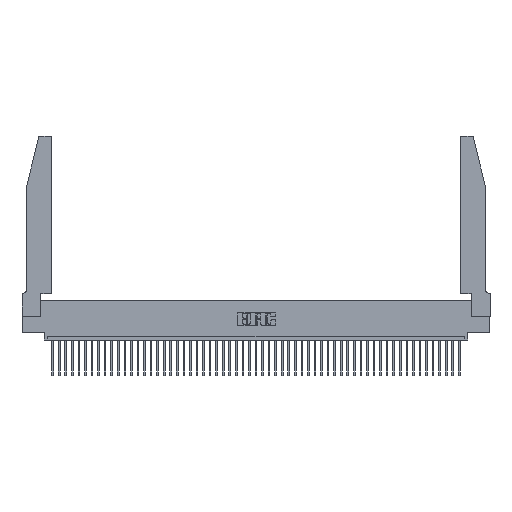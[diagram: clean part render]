
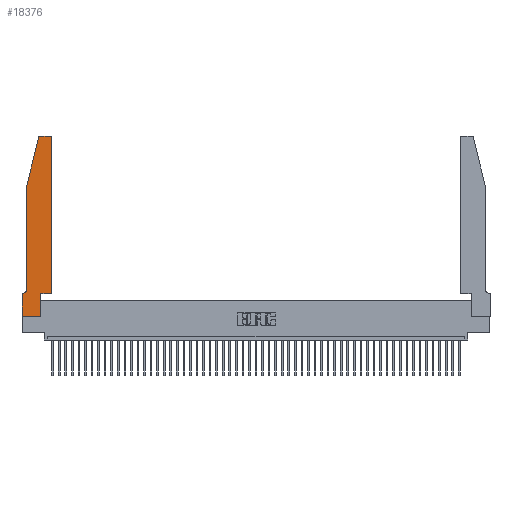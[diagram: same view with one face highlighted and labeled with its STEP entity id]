
A CAD part, top view. The second image highlights one B-rep face of the part: STEP entity #18376.
In plain terms, the highlighted planar face has unit normal (0, 0, 1).
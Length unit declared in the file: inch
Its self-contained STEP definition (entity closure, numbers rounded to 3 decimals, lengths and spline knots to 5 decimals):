
#1313 = CARTESIAN_POINT ( 'NONE',  ( 0., 0.35, 0.37 ) ) ;
#1810 = EDGE_CURVE ( 'NONE', #25819, #5328, #14902, .T. ) ;
#2157 = EDGE_CURVE ( 'NONE', #11748, #25819, #37643, .T. ) ;
#2160 = VERTEX_POINT ( 'NONE', #19044 ) ;
#2213 = DIRECTION ( 'NONE',  ( 0., 0., 1. ) ) ;
#2290 = VERTEX_POINT ( 'NONE', #41261 ) ;
#4435 = ORIENTED_EDGE ( 'NONE', *, *, #1810, .T. ) ;
#4740 = CARTESIAN_POINT ( 'NONE',  ( 0.2865, 0.35, 0.37 ) ) ;
#4752 = EDGE_CURVE ( 'NONE', #5328, #10539, #19771, .T. ) ;
#5328 = VERTEX_POINT ( 'NONE', #38179 ) ;
#6679 = VERTEX_POINT ( 'NONE', #37311 ) ;
#6728 = CARTESIAN_POINT ( 'NONE',  ( 0.2605, 2.75, 0.37 ) ) ;
#8480 = VECTOR ( 'NONE', #44364, 39.37008 ) ;
#10539 = VERTEX_POINT ( 'NONE', #28882 ) ;
#11487 = LINE ( 'NONE', #6728, #8480 ) ;
#11748 = VERTEX_POINT ( 'NONE', #36923 ) ;
#12286 = LINE ( 'NONE', #16870, #24339 ) ;
#14685 = DIRECTION ( 'NONE',  ( -0.239, -0.971, 0. ) ) ;
#14902 = LINE ( 'NONE', #41877, #27407 ) ;
#15348 = LINE ( 'NONE', #37574, #49474 ) ;
#15479 = LINE ( 'NONE', #44176, #34599 ) ;
#15792 = ORIENTED_EDGE ( 'NONE', *, *, #36823, .T. ) ;
#16306 = ORIENTED_EDGE ( 'NONE', *, *, #4752, .T. ) ;
#16452 = DIRECTION ( 'NONE',  ( 0., 1., 0. ) ) ;
#16468 = EDGE_CURVE ( 'NONE', #22883, #6679, #15479, .T. ) ;
#16870 = CARTESIAN_POINT ( 'NONE',  ( 0., 0., 0.37 ) ) ;
#17143 = CARTESIAN_POINT ( 'NONE',  ( 0.25487, 2.72718, 0.37 ) ) ;
#17280 = VECTOR ( 'NONE', #19989, 39.37008 ) ;
#17398 = CARTESIAN_POINT ( 'NONE',  ( 0.4205, 2.72, 0.37 ) ) ;
#17597 = CARTESIAN_POINT ( 'NONE',  ( 0.284, 2.72, 0.37 ) ) ;
#17662 = EDGE_CURVE ( 'NONE', #6679, #36942, #12286, .T. ) ;
#18090 = ORIENTED_EDGE ( 'NONE', *, *, #42210, .T. ) ;
#18376 = ADVANCED_FACE ( 'NONE', ( #35537 ), #47103, .T. ) ;
#19044 = CARTESIAN_POINT ( 'NONE',  ( 0.0755, 0.42, 0.37 ) ) ;
#19212 = DIRECTION ( 'NONE',  ( 1., 0., 0. ) ) ;
#19771 = CIRCLE ( 'NONE', #30226, 0.03 ) ;
#19989 = DIRECTION ( 'NONE',  ( 1., 0., 0. ) ) ;
#21106 = CIRCLE ( 'NONE', #31082, 0.03 ) ;
#22883 = VERTEX_POINT ( 'NONE', #32739 ) ;
#24339 = VECTOR ( 'NONE', #31895, 39.37008 ) ;
#25405 = LINE ( 'NONE', #4740, #28930 ) ;
#25819 = VERTEX_POINT ( 'NONE', #31106 ) ;
#26046 = EDGE_CURVE ( 'NONE', #44971, #11748, #25405, .T. ) ;
#27407 = VECTOR ( 'NONE', #37679, 39.37008 ) ;
#27871 = VECTOR ( 'NONE', #19212, 39.37008 ) ;
#28024 = DIRECTION ( 'NONE',  ( 0., -1., 0. ) ) ;
#28882 = CARTESIAN_POINT ( 'NONE',  ( 0.4205, 2.75, 0.37 ) ) ;
#28930 = VECTOR ( 'NONE', #16452, 39.37008 ) ;
#29595 = DIRECTION ( 'NONE',  ( 0., 0., 1. ) ) ;
#30226 = AXIS2_PLACEMENT_3D ( 'NONE', #17398, #32422, #43829 ) ;
#31082 = AXIS2_PLACEMENT_3D ( 'NONE', #17597, #2213, #48682 ) ;
#31106 = CARTESIAN_POINT ( 'NONE',  ( 0.4505, 0.35, 0.37 ) ) ;
#31321 = ORIENTED_EDGE ( 'NONE', *, *, #26046, .T. ) ;
#31345 = CARTESIAN_POINT ( 'NONE',  ( 0., 0., 0.37 ) ) ;
#31674 = CARTESIAN_POINT ( 'NONE',  ( 0.0755, 2., 0.37 ) ) ;
#31720 = EDGE_CURVE ( 'NONE', #48642, #2290, #15348, .T. ) ;
#31895 = DIRECTION ( 'NONE',  ( 0., -1., 0. ) ) ;
#32064 = DIRECTION ( 'NONE',  ( 0., 0., -1. ) ) ;
#32422 = DIRECTION ( 'NONE',  ( 0., 0., 1. ) ) ;
#32739 = CARTESIAN_POINT ( 'NONE',  ( 0.0055, 0.35, 0.37 ) ) ;
#33336 = CARTESIAN_POINT ( 'NONE',  ( 0.2865, 0., 0.37 ) ) ;
#34599 = VECTOR ( 'NONE', #48660, 39.37008 ) ;
#34962 = ORIENTED_EDGE ( 'NONE', *, *, #2157, .T. ) ;
#35537 = FACE_OUTER_BOUND ( 'NONE', #44798, .T. ) ;
#35626 = VERTEX_POINT ( 'NONE', #37879 ) ;
#36823 = EDGE_CURVE ( 'NONE', #36942, #44971, #36877, .T. ) ;
#36877 = LINE ( 'NONE', #38264, #27871 ) ;
#36923 = CARTESIAN_POINT ( 'NONE',  ( 0.2865, 0.35, 0.37 ) ) ;
#36942 = VERTEX_POINT ( 'NONE', #31345 ) ;
#37311 = CARTESIAN_POINT ( 'NONE',  ( 0., 0.35, 0.37 ) ) ;
#37574 = CARTESIAN_POINT ( 'NONE',  ( 0.0755, 2., 0.37 ) ) ;
#37643 = LINE ( 'NONE', #38260, #17280 ) ;
#37679 = DIRECTION ( 'NONE',  ( 0., 1., 0. ) ) ;
#37799 = AXIS2_PLACEMENT_3D ( 'NONE', #39275, #32064, #43635 ) ;
#37879 = CARTESIAN_POINT ( 'NONE',  ( 0.284, 2.75, 0.37 ) ) ;
#38179 = CARTESIAN_POINT ( 'NONE',  ( 0.4505, 2.72, 0.37 ) ) ;
#38260 = CARTESIAN_POINT ( 'NONE',  ( 0.4505, 0.35, 0.37 ) ) ;
#38264 = CARTESIAN_POINT ( 'NONE',  ( 0., 0., 0.37 ) ) ;
#39275 = CARTESIAN_POINT ( 'NONE',  ( 0.0055, 0.42, 0.37 ) ) ;
#39565 = ORIENTED_EDGE ( 'NONE', *, *, #43577, .T. ) ;
#39697 = LINE ( 'NONE', #31674, #40945 ) ;
#40945 = VECTOR ( 'NONE', #28024, 39.37008 ) ;
#41261 = CARTESIAN_POINT ( 'NONE',  ( 0.0755, 2., 0.37 ) ) ;
#41525 = EDGE_CURVE ( 'NONE', #2160, #22883, #46942, .T. ) ;
#41877 = CARTESIAN_POINT ( 'NONE',  ( 0.4505, 0.35, 0.37 ) ) ;
#42210 = EDGE_CURVE ( 'NONE', #2290, #2160, #39697, .T. ) ;
#42669 = ORIENTED_EDGE ( 'NONE', *, *, #43488, .T. ) ;
#42748 = ORIENTED_EDGE ( 'NONE', *, *, #41525, .T. ) ;
#43488 = EDGE_CURVE ( 'NONE', #35626, #48642, #21106, .T. ) ;
#43577 = EDGE_CURVE ( 'NONE', #10539, #35626, #11487, .T. ) ;
#43635 = DIRECTION ( 'NONE',  ( -1., 0., 0. ) ) ;
#43829 = DIRECTION ( 'NONE',  ( 1., 0., 0. ) ) ;
#44176 = CARTESIAN_POINT ( 'NONE',  ( 0.0755, 0.35, 0.37 ) ) ;
#44364 = DIRECTION ( 'NONE',  ( -1., 0., 0. ) ) ;
#44798 = EDGE_LOOP ( 'NONE', ( #39565, #42669, #47199, #18090, #42748, #47619, #45052, #15792, #31321, #34962, #4435, #16306 ) ) ;
#44971 = VERTEX_POINT ( 'NONE', #33336 ) ;
#45052 = ORIENTED_EDGE ( 'NONE', *, *, #17662, .T. ) ;
#46942 = CIRCLE ( 'NONE', #37799, 0.07 ) ;
#47103 = PLANE ( 'NONE',  #49469 ) ;
#47199 = ORIENTED_EDGE ( 'NONE', *, *, #31720, .T. ) ;
#47381 = DIRECTION ( 'NONE',  ( 1., 0., 0. ) ) ;
#47619 = ORIENTED_EDGE ( 'NONE', *, *, #16468, .T. ) ;
#48642 = VERTEX_POINT ( 'NONE', #17143 ) ;
#48660 = DIRECTION ( 'NONE',  ( -1., 0., 0. ) ) ;
#48682 = DIRECTION ( 'NONE',  ( 1., 0., 0. ) ) ;
#49469 = AXIS2_PLACEMENT_3D ( 'NONE', #1313, #29595, #47381 ) ;
#49474 = VECTOR ( 'NONE', #14685, 39.37008 ) ;
